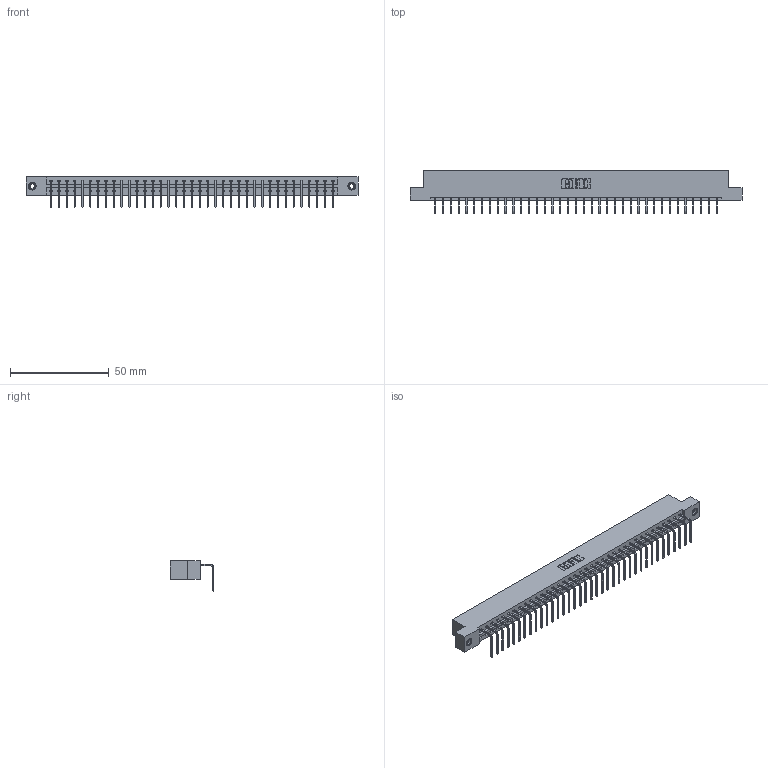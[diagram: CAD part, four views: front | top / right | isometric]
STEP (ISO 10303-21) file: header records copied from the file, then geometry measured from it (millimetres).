
FILE_DESCRIPTION (( 'STEP AP203' ), '1' );
FILE_NAME ('833-037-558-108.STEP', '2020-06-03T05:46:08', ( '' ), ( '' ), 'SwSTEP 2.0', 'SolidWorks 2020', '' );
FILE_SCHEMA (( 'CONFIG_CONTROL_DESIGN' ));
Length unit declared in the file: inch
Products named in the file (4): 345-292-001_558 Tail - 2; 833-037-558-108; 345-250-001_345-250-003-102; 833 Part_Flush - .156 Dia - TI
Assembly tree (40 placements, depth 2):
  833-037-558-108
    833 Part_Flush - .156 Dia - TI
    345-292-001_558 Tail - 2  x37
    345-250-001_345-250-003-102  x2
Bounding box: 168.15 x 22.17 x 15.37 mm (x, y, z)
Volume: 16994.2 mm3; surface area: 19136.5 mm2
Topology: 40 solids, 40 shells, 2394 faces, 7181 edges, 4730 vertices
Faces by surface type: plane 1730, cylinder 648, cone 12, torus 4
Entity records: 24536 total; most frequent: CARTESIAN_POINT 4216, ORIENTED_EDGE 4182, DIRECTION 3599, EDGE_CURVE 2091, LINE 1943, VECTOR 1943, VERTEX_POINT 1388, AXIS2_PLACEMENT_3D 828
